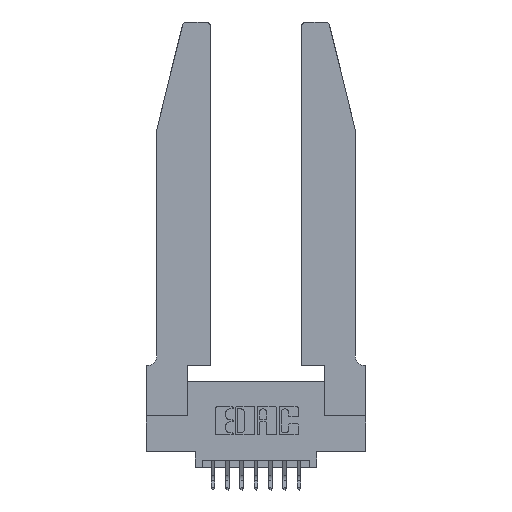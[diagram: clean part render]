
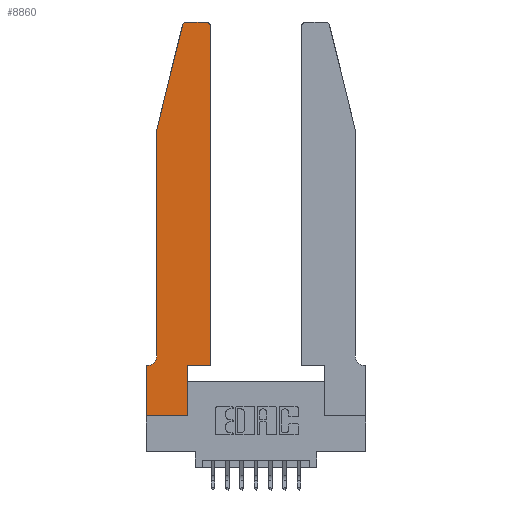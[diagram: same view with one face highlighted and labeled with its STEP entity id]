
A CAD part, top view. The second image highlights one B-rep face of the part: STEP entity #8860.
In plain terms, the highlighted planar face has unit normal (0, 0, 1).
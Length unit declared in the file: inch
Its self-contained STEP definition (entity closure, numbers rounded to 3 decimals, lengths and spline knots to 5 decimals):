
#406 = AXIS2_PLACEMENT_3D ( 'NONE', #3730, #13180, #6103 ) ;
#582 = DIRECTION ( 'NONE',  ( 0., 0., 1. ) ) ;
#663 = VECTOR ( 'NONE', #3564, 39.37008 ) ;
#675 = VECTOR ( 'NONE', #7104, 39.37008 ) ;
#705 = VERTEX_POINT ( 'NONE', #1329 ) ;
#1029 = EDGE_CURVE ( 'NONE', #705, #11019, #4607, .T. ) ;
#1053 = VERTEX_POINT ( 'NONE', #13054 ) ;
#1163 = EDGE_CURVE ( 'NONE', #1053, #12128, #15280, .T. ) ;
#1234 = CARTESIAN_POINT ( 'NONE',  ( 0.4505, 0.35, 0.37 ) ) ;
#1329 = CARTESIAN_POINT ( 'NONE',  ( 0.25487, 2.72718, 0.37 ) ) ;
#1405 = CARTESIAN_POINT ( 'NONE',  ( 0., 0., 0.37 ) ) ;
#1432 = VECTOR ( 'NONE', #12132, 39.37008 ) ;
#1488 = VERTEX_POINT ( 'NONE', #2053 ) ;
#1551 = VERTEX_POINT ( 'NONE', #5765 ) ;
#1834 = VERTEX_POINT ( 'NONE', #7118 ) ;
#2053 = CARTESIAN_POINT ( 'NONE',  ( 0., 0.35, 0.37 ) ) ;
#2085 = CARTESIAN_POINT ( 'NONE',  ( 0.2865, 0., 0.37 ) ) ;
#2179 = CARTESIAN_POINT ( 'NONE',  ( 0.0055, 0.35, 0.37 ) ) ;
#2491 = AXIS2_PLACEMENT_3D ( 'NONE', #3142, #11412, #4342 ) ;
#2553 = PLANE ( 'NONE',  #406 ) ;
#2581 = LINE ( 'NONE', #9766, #15091 ) ;
#2687 = DIRECTION ( 'NONE',  ( 0., -1., 0. ) ) ;
#2908 = ORIENTED_EDGE ( 'NONE', *, *, #5465, .T. ) ;
#3142 = CARTESIAN_POINT ( 'NONE',  ( 0.0055, 0.42, 0.37 ) ) ;
#3564 = DIRECTION ( 'NONE',  ( 1., 0., 0. ) ) ;
#3588 = LINE ( 'NONE', #13669, #12647 ) ;
#3691 = VECTOR ( 'NONE', #13753, 39.37008 ) ;
#3730 = CARTESIAN_POINT ( 'NONE',  ( 0., 0.35, 0.37 ) ) ;
#3809 = ORIENTED_EDGE ( 'NONE', *, *, #10495, .T. ) ;
#4081 = CARTESIAN_POINT ( 'NONE',  ( 0.0755, 0.35, 0.37 ) ) ;
#4144 = CARTESIAN_POINT ( 'NONE',  ( 0.4205, 2.72, 0.37 ) ) ;
#4159 = EDGE_CURVE ( 'NONE', #1551, #705, #7808, .T. ) ;
#4238 = LINE ( 'NONE', #1234, #675 ) ;
#4275 = DIRECTION ( 'NONE',  ( 1., 0., 0. ) ) ;
#4342 = DIRECTION ( 'NONE',  ( -1., 0., 0. ) ) ;
#4432 = LINE ( 'NONE', #11401, #3691 ) ;
#4607 = LINE ( 'NONE', #12905, #1432 ) ;
#4612 = EDGE_CURVE ( 'NONE', #12128, #1551, #3588, .T. ) ;
#4710 = CARTESIAN_POINT ( 'NONE',  ( 0., 0., 0.37 ) ) ;
#4846 = EDGE_CURVE ( 'NONE', #11019, #7221, #11477, .T. ) ;
#5314 = ORIENTED_EDGE ( 'NONE', *, *, #4846, .T. ) ;
#5465 = EDGE_CURVE ( 'NONE', #8666, #10555, #4432, .T. ) ;
#5487 = ORIENTED_EDGE ( 'NONE', *, *, #1029, .T. ) ;
#5668 = EDGE_CURVE ( 'NONE', #1834, #1053, #4238, .T. ) ;
#5765 = CARTESIAN_POINT ( 'NONE',  ( 0.284, 2.75, 0.37 ) ) ;
#6026 = VECTOR ( 'NONE', #7278, 39.37008 ) ;
#6090 = EDGE_LOOP ( 'NONE', ( #15244, #8288, #5487, #5314, #3809, #14698, #6767, #10839, #2908, #13961, #11221, #8698 ) ) ;
#6103 = DIRECTION ( 'NONE',  ( 1., 0., 0. ) ) ;
#6767 = ORIENTED_EDGE ( 'NONE', *, *, #6789, .T. ) ;
#6789 = EDGE_CURVE ( 'NONE', #1488, #7644, #2581, .T. ) ;
#6985 = DIRECTION ( 'NONE',  ( 0., 0., 1. ) ) ;
#6992 = LINE ( 'NONE', #4710, #663 ) ;
#7104 = DIRECTION ( 'NONE',  ( 0., 1., 0. ) ) ;
#7118 = CARTESIAN_POINT ( 'NONE',  ( 0.4505, 0.35, 0.37 ) ) ;
#7221 = VERTEX_POINT ( 'NONE', #14061 ) ;
#7237 = FACE_OUTER_BOUND ( 'NONE', #6090, .T. ) ;
#7278 = DIRECTION ( 'NONE',  ( 1., 0., 0. ) ) ;
#7465 = VECTOR ( 'NONE', #11164, 39.37008 ) ;
#7644 = VERTEX_POINT ( 'NONE', #1405 ) ;
#7808 = CIRCLE ( 'NONE', #14350, 0.03 ) ;
#7870 = DIRECTION ( 'NONE',  ( 0., -1., 0. ) ) ;
#8288 = ORIENTED_EDGE ( 'NONE', *, *, #4159, .T. ) ;
#8449 = LINE ( 'NONE', #13117, #6026 ) ;
#8505 = CIRCLE ( 'NONE', #2491, 0.07 ) ;
#8666 = VERTEX_POINT ( 'NONE', #2085 ) ;
#8698 = ORIENTED_EDGE ( 'NONE', *, *, #1163, .T. ) ;
#8860 = ADVANCED_FACE ( 'NONE', ( #7237 ), #2553, .T. ) ;
#8943 = CARTESIAN_POINT ( 'NONE',  ( 0.0755, 2., 0.37 ) ) ;
#9766 = CARTESIAN_POINT ( 'NONE',  ( 0., 0., 0.37 ) ) ;
#10495 = EDGE_CURVE ( 'NONE', #7221, #13738, #8505, .T. ) ;
#10555 = VERTEX_POINT ( 'NONE', #11467 ) ;
#10650 = EDGE_CURVE ( 'NONE', #7644, #8666, #6992, .T. ) ;
#10839 = ORIENTED_EDGE ( 'NONE', *, *, #10650, .T. ) ;
#11019 = VERTEX_POINT ( 'NONE', #8943 ) ;
#11055 = CARTESIAN_POINT ( 'NONE',  ( 0.4205, 2.75, 0.37 ) ) ;
#11164 = DIRECTION ( 'NONE',  ( -1., 0., 0. ) ) ;
#11221 = ORIENTED_EDGE ( 'NONE', *, *, #5668, .T. ) ;
#11401 = CARTESIAN_POINT ( 'NONE',  ( 0.2865, 0.35, 0.37 ) ) ;
#11412 = DIRECTION ( 'NONE',  ( 0., 0., -1. ) ) ;
#11467 = CARTESIAN_POINT ( 'NONE',  ( 0.2865, 0.35, 0.37 ) ) ;
#11477 = LINE ( 'NONE', #14878, #11865 ) ;
#11865 = VECTOR ( 'NONE', #7870, 39.37008 ) ;
#12128 = VERTEX_POINT ( 'NONE', #11055 ) ;
#12132 = DIRECTION ( 'NONE',  ( -0.239, -0.971, 0. ) ) ;
#12518 = DIRECTION ( 'NONE',  ( -1., 0., 0. ) ) ;
#12531 = EDGE_CURVE ( 'NONE', #10555, #1834, #8449, .T. ) ;
#12647 = VECTOR ( 'NONE', #12518, 39.37008 ) ;
#12905 = CARTESIAN_POINT ( 'NONE',  ( 0.0755, 2., 0.37 ) ) ;
#13054 = CARTESIAN_POINT ( 'NONE',  ( 0.4505, 2.72, 0.37 ) ) ;
#13117 = CARTESIAN_POINT ( 'NONE',  ( 0.4505, 0.35, 0.37 ) ) ;
#13180 = DIRECTION ( 'NONE',  ( 0., 0., 1. ) ) ;
#13627 = AXIS2_PLACEMENT_3D ( 'NONE', #4144, #582, #4275 ) ;
#13669 = CARTESIAN_POINT ( 'NONE',  ( 0.2605, 2.75, 0.37 ) ) ;
#13725 = LINE ( 'NONE', #4081, #7465 ) ;
#13738 = VERTEX_POINT ( 'NONE', #2179 ) ;
#13753 = DIRECTION ( 'NONE',  ( 0., 1., 0. ) ) ;
#13961 = ORIENTED_EDGE ( 'NONE', *, *, #12531, .T. ) ;
#14047 = CARTESIAN_POINT ( 'NONE',  ( 0.284, 2.72, 0.37 ) ) ;
#14061 = CARTESIAN_POINT ( 'NONE',  ( 0.0755, 0.42, 0.37 ) ) ;
#14350 = AXIS2_PLACEMENT_3D ( 'NONE', #14047, #6985, #15224 ) ;
#14698 = ORIENTED_EDGE ( 'NONE', *, *, #15256, .T. ) ;
#14878 = CARTESIAN_POINT ( 'NONE',  ( 0.0755, 2., 0.37 ) ) ;
#15091 = VECTOR ( 'NONE', #2687, 39.37008 ) ;
#15224 = DIRECTION ( 'NONE',  ( 1., 0., 0. ) ) ;
#15244 = ORIENTED_EDGE ( 'NONE', *, *, #4612, .T. ) ;
#15256 = EDGE_CURVE ( 'NONE', #13738, #1488, #13725, .T. ) ;
#15280 = CIRCLE ( 'NONE', #13627, 0.03 ) ;
